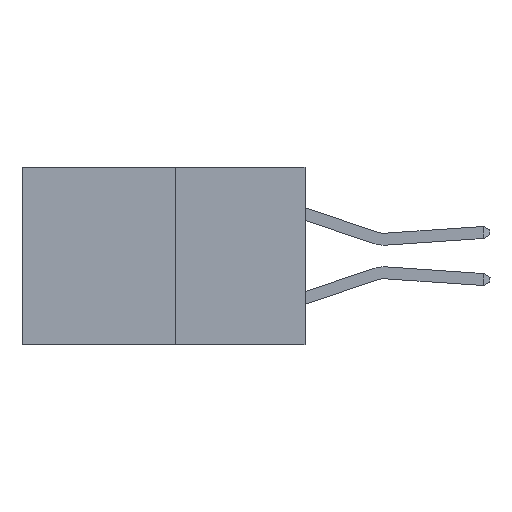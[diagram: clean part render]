
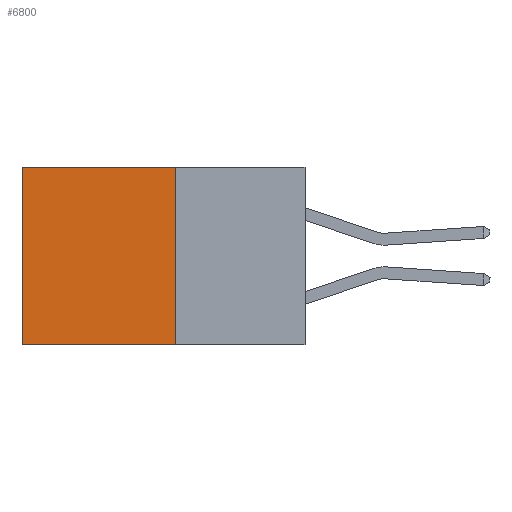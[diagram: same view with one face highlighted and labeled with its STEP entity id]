
A CAD part, left-side view. The second image highlights one B-rep face of the part: STEP entity #6800.
In plain terms, the highlighted planar face has unit normal (-1, 0, 0).
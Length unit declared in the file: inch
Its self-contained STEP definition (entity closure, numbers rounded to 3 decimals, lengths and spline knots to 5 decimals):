
#417 = VECTOR ( 'NONE', #5985, 39.37008 ) ;
#1231 = CARTESIAN_POINT ( 'NONE',  ( 0.277, 0.27, -0.37 ) ) ;
#1235 = ORIENTED_EDGE ( 'NONE', *, *, #3700, .F. ) ;
#1295 = LINE ( 'NONE', #7539, #1553 ) ;
#1504 = VERTEX_POINT ( 'NONE', #1231 ) ;
#1553 = VECTOR ( 'NONE', #5198, 39.37008 ) ;
#2423 = VERTEX_POINT ( 'NONE', #7243 ) ;
#3027 = DIRECTION ( 'NONE',  ( 0., 1., 0. ) ) ;
#3700 = EDGE_CURVE ( 'NONE', #1504, #8359, #7209, .T. ) ;
#3869 = DIRECTION ( 'NONE',  ( 1., 0., 0. ) ) ;
#3905 = EDGE_CURVE ( 'NONE', #5217, #8359, #1295, .T. ) ;
#4377 = LINE ( 'NONE', #9352, #417 ) ;
#4850 = CARTESIAN_POINT ( 'NONE',  ( 0.277, 0.27, -0.37 ) ) ;
#5198 = DIRECTION ( 'NONE',  ( 0., 0., -1. ) ) ;
#5217 = VERTEX_POINT ( 'NONE', #7480 ) ;
#5303 = VECTOR ( 'NONE', #3027, 39.37008 ) ;
#5985 = DIRECTION ( 'NONE',  ( 0., 1., 0. ) ) ;
#6229 = ORIENTED_EDGE ( 'NONE', *, *, #3905, .T. ) ;
#6800 = ADVANCED_FACE ( 'NONE', ( #8722 ), #6827, .F. ) ;
#6827 = PLANE ( 'NONE',  #7255 ) ;
#7209 = LINE ( 'NONE', #9147, #5303 ) ;
#7243 = CARTESIAN_POINT ( 'NONE',  ( 0.277, 0.27, 0. ) ) ;
#7255 = AXIS2_PLACEMENT_3D ( 'NONE', #8815, #3869, #8840 ) ;
#7320 = VECTOR ( 'NONE', #7717, 39.37008 ) ;
#7480 = CARTESIAN_POINT ( 'NONE',  ( 0.277, 0.59, 0. ) ) ;
#7539 = CARTESIAN_POINT ( 'NONE',  ( 0.277, 0.59, -0.37 ) ) ;
#7717 = DIRECTION ( 'NONE',  ( 0., 0., -1. ) ) ;
#7767 = CARTESIAN_POINT ( 'NONE',  ( 0.277, 0.59, -0.37 ) ) ;
#8359 = VERTEX_POINT ( 'NONE', #7767 ) ;
#8690 = ORIENTED_EDGE ( 'NONE', *, *, #9069, .F. ) ;
#8722 = FACE_OUTER_BOUND ( 'NONE', #9028, .T. ) ;
#8815 = CARTESIAN_POINT ( 'NONE',  ( 0.277, 0.27, -0.37 ) ) ;
#8840 = DIRECTION ( 'NONE',  ( 0., 0., -1. ) ) ;
#9028 = EDGE_LOOP ( 'NONE', ( #6229, #1235, #8690, #9335 ) ) ;
#9069 = EDGE_CURVE ( 'NONE', #2423, #1504, #9100, .T. ) ;
#9100 = LINE ( 'NONE', #4850, #7320 ) ;
#9147 = CARTESIAN_POINT ( 'NONE',  ( 0.277, 0.27, -0.37 ) ) ;
#9335 = ORIENTED_EDGE ( 'NONE', *, *, #9409, .T. ) ;
#9352 = CARTESIAN_POINT ( 'NONE',  ( 0.277, 0.27, 0. ) ) ;
#9409 = EDGE_CURVE ( 'NONE', #2423, #5217, #4377, .T. ) ;
